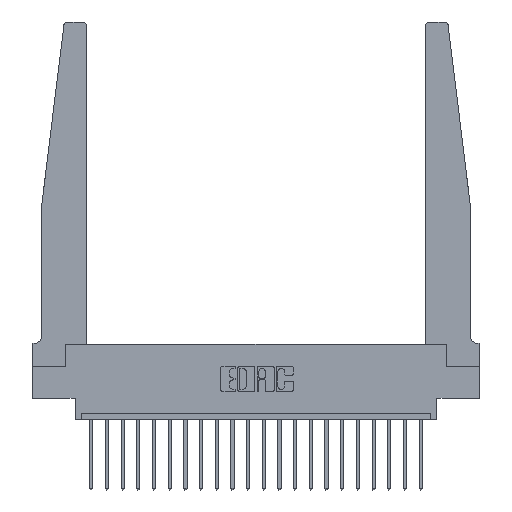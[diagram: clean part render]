
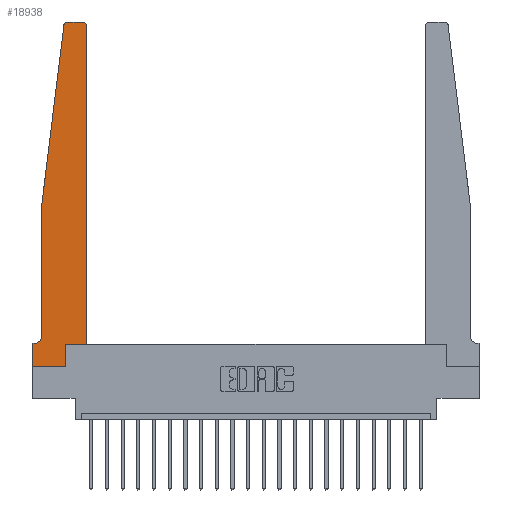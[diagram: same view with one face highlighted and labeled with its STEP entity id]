
A CAD part, top view. The second image highlights one B-rep face of the part: STEP entity #18938.
In plain terms, the highlighted planar face has unit normal (0, 0, 1).
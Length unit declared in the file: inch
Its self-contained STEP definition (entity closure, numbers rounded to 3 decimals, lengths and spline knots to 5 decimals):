
#203 = CIRCLE ( 'NONE', #14555, 0.05 ) ;
#275 = VECTOR ( 'NONE', #444, 39.37008 ) ;
#444 = DIRECTION ( 'NONE',  ( -1., 0., 0. ) ) ;
#480 = VERTEX_POINT ( 'NONE', #21345 ) ;
#1177 = DIRECTION ( 'NONE',  ( 0., 1., 0. ) ) ;
#1559 = AXIS2_PLACEMENT_3D ( 'NONE', #5094, #21460, #8393 ) ;
#1770 = CARTESIAN_POINT ( 'NONE',  ( 0.25, 2.75, 0.37 ) ) ;
#1897 = CARTESIAN_POINT ( 'NONE',  ( 0.27653, 2.72, 0.37 ) ) ;
#2048 = VERTEX_POINT ( 'NONE', #14211 ) ;
#2665 = EDGE_CURVE ( 'NONE', #16450, #10846, #13830, .T. ) ;
#2768 = LINE ( 'NONE', #9223, #21234 ) ;
#2962 = DIRECTION ( 'NONE',  ( 1., 0., 0. ) ) ;
#3212 = DIRECTION ( 'NONE',  ( 0., 0., -1. ) ) ;
#3347 = DIRECTION ( 'NONE',  ( 0., 0., 1. ) ) ;
#3422 = VECTOR ( 'NONE', #13862, 39.37008 ) ;
#3637 = CARTESIAN_POINT ( 'NONE',  ( 0.425, 0.18, 0.37 ) ) ;
#3746 = EDGE_CURVE ( 'NONE', #7250, #15155, #18912, .T. ) ;
#3807 = CARTESIAN_POINT ( 'NONE',  ( 0.2605, 0.18, 0.37 ) ) ;
#3881 = DIRECTION ( 'NONE',  ( 0., 1., 0. ) ) ;
#5094 = CARTESIAN_POINT ( 'NONE',  ( 0.395, 2.72, 0.37 ) ) ;
#5264 = ORIENTED_EDGE ( 'NONE', *, *, #19665, .T. ) ;
#6088 = CARTESIAN_POINT ( 'NONE',  ( 0.065, 0.2375, 0.37 ) ) ;
#6319 = LINE ( 'NONE', #16210, #17658 ) ;
#6449 = VERTEX_POINT ( 'NONE', #13869 ) ;
#6563 = EDGE_LOOP ( 'NONE', ( #8685, #7851, #5264, #17974, #19422, #20628, #7097, #6963, #17930, #20290, #14065, #17422 ) ) ;
#6795 = CARTESIAN_POINT ( 'NONE',  ( 0.065, 0.1875, 0.37 ) ) ;
#6799 = VECTOR ( 'NONE', #15409, 39.37008 ) ;
#6963 = ORIENTED_EDGE ( 'NONE', *, *, #13215, .T. ) ;
#7097 = ORIENTED_EDGE ( 'NONE', *, *, #12768, .T. ) ;
#7250 = VERTEX_POINT ( 'NONE', #3807 ) ;
#7367 = VERTEX_POINT ( 'NONE', #6088 ) ;
#7506 = CIRCLE ( 'NONE', #1559, 0.03 ) ;
#7851 = ORIENTED_EDGE ( 'NONE', *, *, #15104, .T. ) ;
#7984 = DIRECTION ( 'NONE',  ( 0., -1., 0. ) ) ;
#8393 = DIRECTION ( 'NONE',  ( 1., 0., 0. ) ) ;
#8445 = LINE ( 'NONE', #18213, #10677 ) ;
#8685 = ORIENTED_EDGE ( 'NONE', *, *, #2665, .T. ) ;
#8702 = EDGE_CURVE ( 'NONE', #6449, #7367, #16550, .T. ) ;
#8711 = CARTESIAN_POINT ( 'NONE',  ( 0., 0., 0.37 ) ) ;
#9223 = CARTESIAN_POINT ( 'NONE',  ( 0.065, 1.25, 0.37 ) ) ;
#9891 = DIRECTION ( 'NONE',  ( -1., 0., 0. ) ) ;
#10216 = DIRECTION ( 'NONE',  ( -1., 0., 0. ) ) ;
#10349 = VERTEX_POINT ( 'NONE', #17982 ) ;
#10569 = CARTESIAN_POINT ( 'NONE',  ( 0.425, 0.18, 0.37 ) ) ;
#10646 = VERTEX_POINT ( 'NONE', #10849 ) ;
#10677 = VECTOR ( 'NONE', #2962, 39.37008 ) ;
#10846 = VERTEX_POINT ( 'NONE', #13353 ) ;
#10849 = CARTESIAN_POINT ( 'NONE',  ( 0.015, 0.1875, 0.37 ) ) ;
#10988 = DIRECTION ( 'NONE',  ( -0.122, -0.992, 0. ) ) ;
#12292 = VECTOR ( 'NONE', #7984, 39.37008 ) ;
#12768 = EDGE_CURVE ( 'NONE', #20336, #480, #21676, .T. ) ;
#12791 = EDGE_CURVE ( 'NONE', #15155, #10349, #15847, .T. ) ;
#13006 = EDGE_CURVE ( 'NONE', #17962, #7250, #6319, .T. ) ;
#13215 = EDGE_CURVE ( 'NONE', #480, #17962, #8445, .T. ) ;
#13230 = DIRECTION ( 'NONE',  ( 1., 0., 0. ) ) ;
#13333 = FACE_OUTER_BOUND ( 'NONE', #6563, .T. ) ;
#13353 = CARTESIAN_POINT ( 'NONE',  ( 0.27653, 2.75, 0.37 ) ) ;
#13553 = AXIS2_PLACEMENT_3D ( 'NONE', #21680, #3347, #13230 ) ;
#13556 = PLANE ( 'NONE',  #13553 ) ;
#13619 = LINE ( 'NONE', #6795, #275 ) ;
#13771 = EDGE_CURVE ( 'NONE', #7367, #10646, #203, .T. ) ;
#13817 = VECTOR ( 'NONE', #3881, 39.37008 ) ;
#13830 = LINE ( 'NONE', #1770, #18106 ) ;
#13862 = DIRECTION ( 'NONE',  ( 1., 0., 0. ) ) ;
#13869 = CARTESIAN_POINT ( 'NONE',  ( 0.065, 1.25, 0.37 ) ) ;
#14065 = ORIENTED_EDGE ( 'NONE', *, *, #12791, .T. ) ;
#14211 = CARTESIAN_POINT ( 'NONE',  ( 0.24675, 2.72367, 0.37 ) ) ;
#14555 = AXIS2_PLACEMENT_3D ( 'NONE', #16268, #3212, #9891 ) ;
#15104 = EDGE_CURVE ( 'NONE', #10846, #2048, #15535, .T. ) ;
#15155 = VERTEX_POINT ( 'NONE', #3637 ) ;
#15409 = DIRECTION ( 'NONE',  ( 0., -1., 0. ) ) ;
#15535 = CIRCLE ( 'NONE', #18347, 0.03 ) ;
#15620 = CARTESIAN_POINT ( 'NONE',  ( 0.425, 0.18, 0.37 ) ) ;
#15847 = LINE ( 'NONE', #15620, #13817 ) ;
#16189 = EDGE_CURVE ( 'NONE', #10349, #16450, #7506, .T. ) ;
#16210 = CARTESIAN_POINT ( 'NONE',  ( 0.2605, 0.18, 0.37 ) ) ;
#16268 = CARTESIAN_POINT ( 'NONE',  ( 0.015, 0.2375, 0.37 ) ) ;
#16330 = CARTESIAN_POINT ( 'NONE',  ( 0.065, 1.25, 0.37 ) ) ;
#16450 = VERTEX_POINT ( 'NONE', #17265 ) ;
#16550 = LINE ( 'NONE', #16330, #12292 ) ;
#16914 = DIRECTION ( 'NONE',  ( 1., 0., 0. ) ) ;
#17265 = CARTESIAN_POINT ( 'NONE',  ( 0.395, 2.75, 0.37 ) ) ;
#17422 = ORIENTED_EDGE ( 'NONE', *, *, #16189, .T. ) ;
#17658 = VECTOR ( 'NONE', #1177, 39.37008 ) ;
#17930 = ORIENTED_EDGE ( 'NONE', *, *, #13006, .T. ) ;
#17962 = VERTEX_POINT ( 'NONE', #18712 ) ;
#17974 = ORIENTED_EDGE ( 'NONE', *, *, #8702, .T. ) ;
#17982 = CARTESIAN_POINT ( 'NONE',  ( 0.425, 2.72, 0.37 ) ) ;
#18106 = VECTOR ( 'NONE', #10216, 39.37008 ) ;
#18213 = CARTESIAN_POINT ( 'NONE',  ( 0., 0., 0.37 ) ) ;
#18250 = DIRECTION ( 'NONE',  ( 0., 0., 1. ) ) ;
#18347 = AXIS2_PLACEMENT_3D ( 'NONE', #1897, #18250, #16914 ) ;
#18712 = CARTESIAN_POINT ( 'NONE',  ( 0.2605, 0., 0.37 ) ) ;
#18912 = LINE ( 'NONE', #10569, #3422 ) ;
#18938 = ADVANCED_FACE ( 'NONE', ( #13333 ), #13556, .T. ) ;
#19422 = ORIENTED_EDGE ( 'NONE', *, *, #13771, .T. ) ;
#19665 = EDGE_CURVE ( 'NONE', #2048, #6449, #2768, .T. ) ;
#20290 = ORIENTED_EDGE ( 'NONE', *, *, #3746, .T. ) ;
#20336 = VERTEX_POINT ( 'NONE', #20366 ) ;
#20366 = CARTESIAN_POINT ( 'NONE',  ( 0., 0.1875, 0.37 ) ) ;
#20628 = ORIENTED_EDGE ( 'NONE', *, *, #21391, .T. ) ;
#21234 = VECTOR ( 'NONE', #10988, 39.37008 ) ;
#21345 = CARTESIAN_POINT ( 'NONE',  ( 0., 0., 0.37 ) ) ;
#21391 = EDGE_CURVE ( 'NONE', #10646, #20336, #13619, .T. ) ;
#21460 = DIRECTION ( 'NONE',  ( 0., 0., 1. ) ) ;
#21676 = LINE ( 'NONE', #8711, #6799 ) ;
#21680 = CARTESIAN_POINT ( 'NONE',  ( 0., 0.1875, 0.37 ) ) ;
